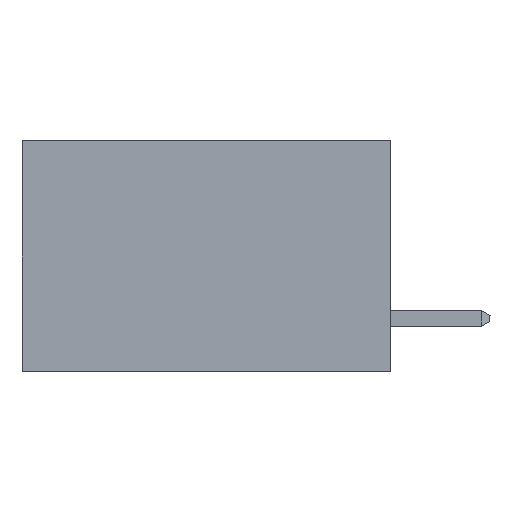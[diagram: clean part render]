
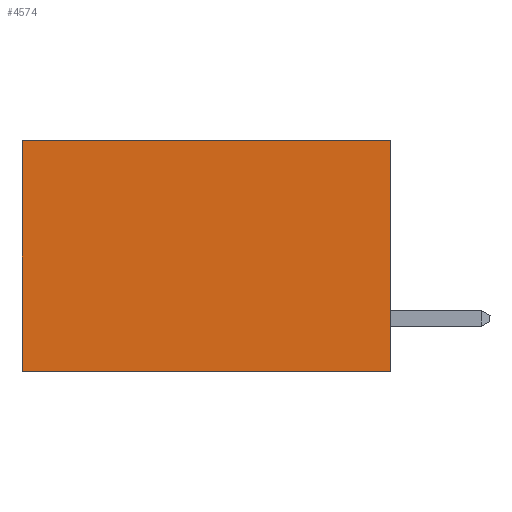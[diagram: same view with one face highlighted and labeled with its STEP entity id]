
A CAD part, left-side view. The second image highlights one B-rep face of the part: STEP entity #4574.
In plain terms, the highlighted planar face has unit normal (-1, 0, 0).
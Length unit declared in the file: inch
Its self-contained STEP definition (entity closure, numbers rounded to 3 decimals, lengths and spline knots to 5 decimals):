
#194 = DIRECTION ( 'NONE',  ( 0., 0., -1. ) ) ;
#263 = DIRECTION ( 'NONE',  ( 1., 0., 0. ) ) ;
#280 = CARTESIAN_POINT ( 'NONE',  ( 0.277, 0., -0.37 ) ) ;
#381 = PLANE ( 'NONE',  #6044 ) ;
#965 = VERTEX_POINT ( 'NONE', #7843 ) ;
#1040 = CARTESIAN_POINT ( 'NONE',  ( 0.277, 0., -0.37 ) ) ;
#1389 = EDGE_CURVE ( 'NONE', #965, #6444, #2759, .T. ) ;
#1420 = DIRECTION ( 'NONE',  ( 0., 1., 0. ) ) ;
#1639 = VECTOR ( 'NONE', #1420, 39.37008 ) ;
#2184 = VECTOR ( 'NONE', #2499, 39.37008 ) ;
#2265 = CARTESIAN_POINT ( 'NONE',  ( 0.277, 0.59, -0.37 ) ) ;
#2499 = DIRECTION ( 'NONE',  ( 0., 1., 0. ) ) ;
#2531 = VECTOR ( 'NONE', #6557, 39.37008 ) ;
#2559 = VERTEX_POINT ( 'NONE', #3323 ) ;
#2759 = LINE ( 'NONE', #5231, #2531 ) ;
#2805 = CARTESIAN_POINT ( 'NONE',  ( 0.277, 0., 0. ) ) ;
#3281 = EDGE_LOOP ( 'NONE', ( #5349, #5581, #7885, #6983 ) ) ;
#3323 = CARTESIAN_POINT ( 'NONE',  ( 0.277, 0.59, 0. ) ) ;
#3981 = LINE ( 'NONE', #2805, #2184 ) ;
#4481 = EDGE_CURVE ( 'NONE', #6444, #8036, #6609, .T. ) ;
#4574 = ADVANCED_FACE ( 'NONE', ( #7743 ), #381, .F. ) ;
#4847 = EDGE_CURVE ( 'NONE', #965, #2559, #3981, .T. ) ;
#5085 = DIRECTION ( 'NONE',  ( 0., 0., -1. ) ) ;
#5231 = CARTESIAN_POINT ( 'NONE',  ( 0.277, 0., -0.37 ) ) ;
#5349 = ORIENTED_EDGE ( 'NONE', *, *, #8542, .T. ) ;
#5581 = ORIENTED_EDGE ( 'NONE', *, *, #4481, .F. ) ;
#6044 = AXIS2_PLACEMENT_3D ( 'NONE', #280, #263, #194 ) ;
#6444 = VERTEX_POINT ( 'NONE', #6453 ) ;
#6447 = CARTESIAN_POINT ( 'NONE',  ( 0.277, 0.59, -0.37 ) ) ;
#6453 = CARTESIAN_POINT ( 'NONE',  ( 0.277, 0., -0.37 ) ) ;
#6557 = DIRECTION ( 'NONE',  ( 0., 0., -1. ) ) ;
#6609 = LINE ( 'NONE', #1040, #1639 ) ;
#6983 = ORIENTED_EDGE ( 'NONE', *, *, #4847, .T. ) ;
#7660 = VECTOR ( 'NONE', #5085, 39.37008 ) ;
#7743 = FACE_OUTER_BOUND ( 'NONE', #3281, .T. ) ;
#7843 = CARTESIAN_POINT ( 'NONE',  ( 0.277, 0., 0. ) ) ;
#7855 = LINE ( 'NONE', #6447, #7660 ) ;
#7885 = ORIENTED_EDGE ( 'NONE', *, *, #1389, .F. ) ;
#8036 = VERTEX_POINT ( 'NONE', #2265 ) ;
#8542 = EDGE_CURVE ( 'NONE', #2559, #8036, #7855, .T. ) ;
